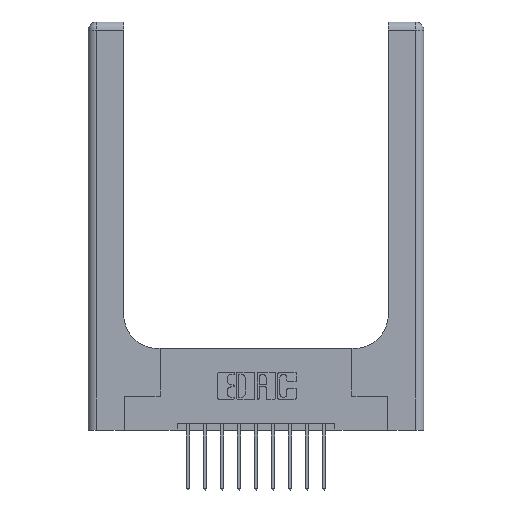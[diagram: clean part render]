
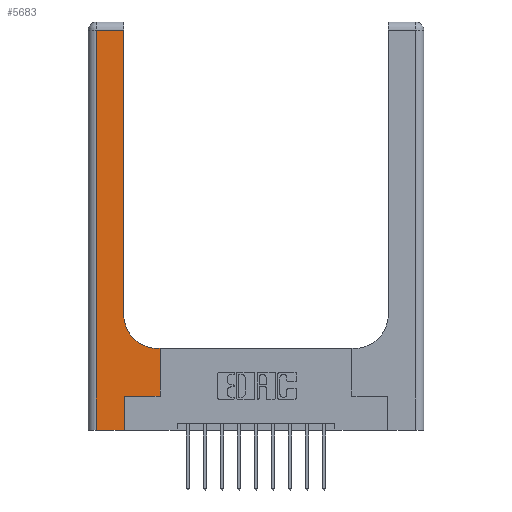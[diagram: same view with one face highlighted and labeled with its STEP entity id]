
A CAD part, top view. The second image highlights one B-rep face of the part: STEP entity #5683.
In plain terms, the highlighted planar face has unit normal (0, 0, 1).
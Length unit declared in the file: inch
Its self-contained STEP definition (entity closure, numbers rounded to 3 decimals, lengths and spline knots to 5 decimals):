
#108 = AXIS2_PLACEMENT_3D ( 'NONE', #10647, #13395, #2332 ) ;
#1034 = CARTESIAN_POINT ( 'NONE',  ( 0.265, 0., 0.37 ) ) ;
#1040 = VECTOR ( 'NONE', #2564, 39.37008 ) ;
#1128 = VERTEX_POINT ( 'NONE', #3519 ) ;
#1152 = CARTESIAN_POINT ( 'NONE',  ( 0.265, 0.25, 0.37 ) ) ;
#1355 = EDGE_CURVE ( 'NONE', #8071, #5921, #4205, .T. ) ;
#1358 = DIRECTION ( 'NONE',  ( 0., 1., 0. ) ) ;
#2171 = CARTESIAN_POINT ( 'NONE',  ( 0.51, 0.85, 0.37 ) ) ;
#2332 = DIRECTION ( 'NONE',  ( -1., 0., 0. ) ) ;
#2410 = DIRECTION ( 'NONE',  ( 0., 1., 0. ) ) ;
#2415 = CARTESIAN_POINT ( 'NONE',  ( 0.26, 2.94, 0.37 ) ) ;
#2481 = EDGE_CURVE ( 'NONE', #12571, #15734, #14186, .T. ) ;
#2564 = DIRECTION ( 'NONE',  ( 0., -1., 0. ) ) ;
#3090 = DIRECTION ( 'NONE',  ( 1., 0., 0. ) ) ;
#3423 = LINE ( 'NONE', #12236, #10159 ) ;
#3446 = FACE_OUTER_BOUND ( 'NONE', #9960, .T. ) ;
#3519 = CARTESIAN_POINT ( 'NONE',  ( 0.265, 0., 0.37 ) ) ;
#3563 = VECTOR ( 'NONE', #2410, 39.37008 ) ;
#3790 = CARTESIAN_POINT ( 'NONE',  ( 0.528, 0.25, 0.37 ) ) ;
#3946 = VERTEX_POINT ( 'NONE', #1152 ) ;
#4147 = CARTESIAN_POINT ( 'NONE',  ( 0.06, 2.94, 0.37 ) ) ;
#4149 = CARTESIAN_POINT ( 'NONE',  ( 0., 0., 0.37 ) ) ;
#4205 = LINE ( 'NONE', #5748, #15805 ) ;
#4223 = VERTEX_POINT ( 'NONE', #9416 ) ;
#4369 = EDGE_CURVE ( 'NONE', #1128, #3946, #15812, .T. ) ;
#4455 = EDGE_CURVE ( 'NONE', #15081, #12571, #3423, .T. ) ;
#4557 = CARTESIAN_POINT ( 'NONE',  ( 0.26, 3., 0.37 ) ) ;
#4788 = DIRECTION ( 'NONE',  ( 0., 1., 0. ) ) ;
#5307 = DIRECTION ( 'NONE',  ( 1., 0., 0. ) ) ;
#5431 = DIRECTION ( 'NONE',  ( -1., 0., 0. ) ) ;
#5553 = DIRECTION ( 'NONE',  ( 0., 0., -1. ) ) ;
#5683 = ADVANCED_FACE ( 'NONE', ( #3446 ), #6927, .F. ) ;
#5697 = VECTOR ( 'NONE', #3090, 39.37008 ) ;
#5748 = CARTESIAN_POINT ( 'NONE',  ( 0., 2.94, 0.37 ) ) ;
#5921 = VERTEX_POINT ( 'NONE', #4147 ) ;
#6033 = VERTEX_POINT ( 'NONE', #3790 ) ;
#6598 = CARTESIAN_POINT ( 'NONE',  ( 0.06, 3., 0.37 ) ) ;
#6826 = VECTOR ( 'NONE', #5307, 39.37008 ) ;
#6927 = PLANE ( 'NONE',  #108 ) ;
#7462 = CARTESIAN_POINT ( 'NONE',  ( 0.528, 0.25, 0.37 ) ) ;
#8071 = VERTEX_POINT ( 'NONE', #2415 ) ;
#8233 = EDGE_CURVE ( 'NONE', #4223, #1128, #15259, .T. ) ;
#8257 = AXIS2_PLACEMENT_3D ( 'NONE', #2171, #5553, #15356 ) ;
#8430 = ORIENTED_EDGE ( 'NONE', *, *, #8233, .T. ) ;
#8540 = LINE ( 'NONE', #4557, #3563 ) ;
#8845 = CARTESIAN_POINT ( 'NONE',  ( 0.26, 0.85, 0.37 ) ) ;
#8871 = VECTOR ( 'NONE', #4788, 39.37008 ) ;
#9027 = LINE ( 'NONE', #6598, #1040 ) ;
#9154 = CARTESIAN_POINT ( 'NONE',  ( 0.265, 0.25, 0.37 ) ) ;
#9416 = CARTESIAN_POINT ( 'NONE',  ( 0.06, 0., 0.37 ) ) ;
#9731 = EDGE_CURVE ( 'NONE', #6033, #15081, #13618, .T. ) ;
#9829 = ORIENTED_EDGE ( 'NONE', *, *, #4369, .T. ) ;
#9864 = ORIENTED_EDGE ( 'NONE', *, *, #4455, .T. ) ;
#9874 = ORIENTED_EDGE ( 'NONE', *, *, #13064, .T. ) ;
#9960 = EDGE_LOOP ( 'NONE', ( #15657, #10105, #9874, #8430, #9829, #13122, #11277, #9864, #10763 ) ) ;
#10105 = ORIENTED_EDGE ( 'NONE', *, *, #1355, .T. ) ;
#10159 = VECTOR ( 'NONE', #12073, 39.37008 ) ;
#10446 = LINE ( 'NONE', #9154, #5697 ) ;
#10647 = CARTESIAN_POINT ( 'NONE',  ( 0., 3., 0.37 ) ) ;
#10763 = ORIENTED_EDGE ( 'NONE', *, *, #2481, .T. ) ;
#11277 = ORIENTED_EDGE ( 'NONE', *, *, #9731, .T. ) ;
#11624 = EDGE_CURVE ( 'NONE', #15734, #8071, #8540, .T. ) ;
#12073 = DIRECTION ( 'NONE',  ( -1., 0., 0. ) ) ;
#12236 = CARTESIAN_POINT ( 'NONE',  ( 0.26, 0.6, 0.37 ) ) ;
#12571 = VERTEX_POINT ( 'NONE', #15121 ) ;
#13064 = EDGE_CURVE ( 'NONE', #5921, #4223, #9027, .T. ) ;
#13122 = ORIENTED_EDGE ( 'NONE', *, *, #14759, .T. ) ;
#13395 = DIRECTION ( 'NONE',  ( 0., 0., -1. ) ) ;
#13618 = LINE ( 'NONE', #7462, #15654 ) ;
#14186 = CIRCLE ( 'NONE', #8257, 0.25 ) ;
#14759 = EDGE_CURVE ( 'NONE', #3946, #6033, #10446, .T. ) ;
#15081 = VERTEX_POINT ( 'NONE', #15736 ) ;
#15121 = CARTESIAN_POINT ( 'NONE',  ( 0.51, 0.6, 0.37 ) ) ;
#15259 = LINE ( 'NONE', #4149, #6826 ) ;
#15356 = DIRECTION ( 'NONE',  ( 1., 0., 0. ) ) ;
#15654 = VECTOR ( 'NONE', #1358, 39.37008 ) ;
#15657 = ORIENTED_EDGE ( 'NONE', *, *, #11624, .T. ) ;
#15734 = VERTEX_POINT ( 'NONE', #8845 ) ;
#15736 = CARTESIAN_POINT ( 'NONE',  ( 0.528, 0.6, 0.37 ) ) ;
#15805 = VECTOR ( 'NONE', #5431, 39.37008 ) ;
#15812 = LINE ( 'NONE', #1034, #8871 ) ;
